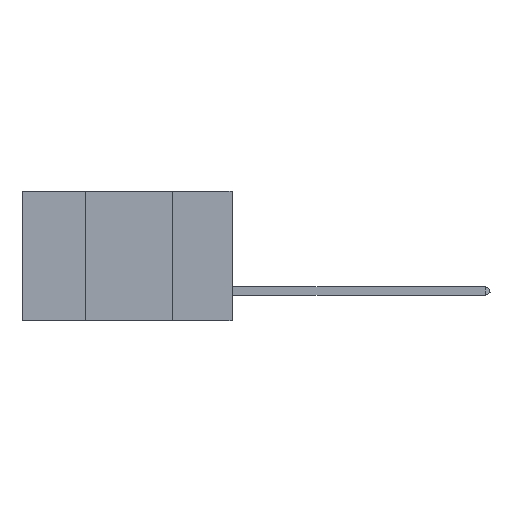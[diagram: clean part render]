
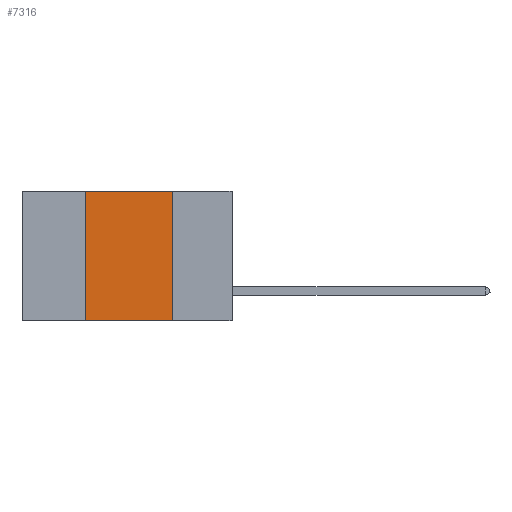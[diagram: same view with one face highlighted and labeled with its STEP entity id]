
A CAD part, left-side view. The second image highlights one B-rep face of the part: STEP entity #7316.
In plain terms, the highlighted planar face has unit normal (-1, 0, 0).
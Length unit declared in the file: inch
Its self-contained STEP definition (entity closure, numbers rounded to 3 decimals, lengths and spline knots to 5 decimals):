
#1759 = PLANE ( 'NONE',  #14349 ) ;
#1918 = CARTESIAN_POINT ( 'NONE',  ( 0., 0.17, 0. ) ) ;
#5514 = DIRECTION ( 'NONE',  ( 0., 0., -1. ) ) ;
#7274 = LINE ( 'NONE', #16730, #38871 ) ;
#7316 = ADVANCED_FACE ( 'NONE', ( #32590 ), #1759, .F. ) ;
#7490 = DIRECTION ( 'NONE',  ( 0., 0., 1. ) ) ;
#9749 = CARTESIAN_POINT ( 'NONE',  ( 0., 0.17, 0. ) ) ;
#11406 = EDGE_CURVE ( 'NONE', #42486, #27605, #18016, .T. ) ;
#12128 = DIRECTION ( 'NONE',  ( 0., -1., 0. ) ) ;
#14349 = AXIS2_PLACEMENT_3D ( 'NONE', #15479, #29451, #29663 ) ;
#14390 = VERTEX_POINT ( 'NONE', #41866 ) ;
#15479 = CARTESIAN_POINT ( 'NONE',  ( 0., 0.6, 0. ) ) ;
#16730 = CARTESIAN_POINT ( 'NONE',  ( 0., 0.42, 0. ) ) ;
#18016 = LINE ( 'NONE', #28388, #28057 ) ;
#19115 = LINE ( 'NONE', #29266, #24477 ) ;
#22615 = LINE ( 'NONE', #1918, #28974 ) ;
#24477 = VECTOR ( 'NONE', #12128, 39.37008 ) ;
#27605 = VERTEX_POINT ( 'NONE', #38645 ) ;
#28057 = VECTOR ( 'NONE', #31746, 39.37008 ) ;
#28388 = CARTESIAN_POINT ( 'NONE',  ( 0., 0.6, -0.37 ) ) ;
#28974 = VECTOR ( 'NONE', #5514, 39.37008 ) ;
#29224 = EDGE_CURVE ( 'NONE', #42486, #14390, #7274, .T. ) ;
#29266 = CARTESIAN_POINT ( 'NONE',  ( 0., 0.6, 0. ) ) ;
#29451 = DIRECTION ( 'NONE',  ( 1., 0., 0. ) ) ;
#29663 = DIRECTION ( 'NONE',  ( 0., 0., -1. ) ) ;
#30674 = ORIENTED_EDGE ( 'NONE', *, *, #11406, .T. ) ;
#30769 = CARTESIAN_POINT ( 'NONE',  ( 0., 0.42, -0.37 ) ) ;
#31746 = DIRECTION ( 'NONE',  ( 0., -1., 0. ) ) ;
#32590 = FACE_OUTER_BOUND ( 'NONE', #41922, .T. ) ;
#33332 = ORIENTED_EDGE ( 'NONE', *, *, #39925, .F. ) ;
#37109 = EDGE_CURVE ( 'NONE', #14390, #38001, #19115, .T. ) ;
#38001 = VERTEX_POINT ( 'NONE', #9749 ) ;
#38645 = CARTESIAN_POINT ( 'NONE',  ( 0., 0.17, -0.37 ) ) ;
#38871 = VECTOR ( 'NONE', #7490, 39.37008 ) ;
#39925 = EDGE_CURVE ( 'NONE', #38001, #27605, #22615, .T. ) ;
#40604 = ORIENTED_EDGE ( 'NONE', *, *, #29224, .F. ) ;
#41737 = ORIENTED_EDGE ( 'NONE', *, *, #37109, .F. ) ;
#41866 = CARTESIAN_POINT ( 'NONE',  ( 0., 0.42, 0. ) ) ;
#41922 = EDGE_LOOP ( 'NONE', ( #33332, #41737, #40604, #30674 ) ) ;
#42486 = VERTEX_POINT ( 'NONE', #30769 ) ;
